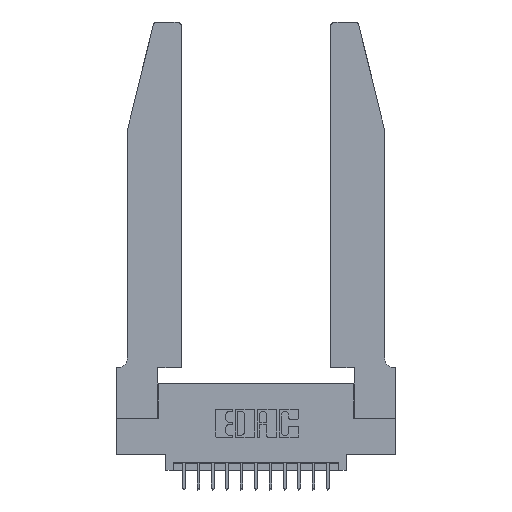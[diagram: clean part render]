
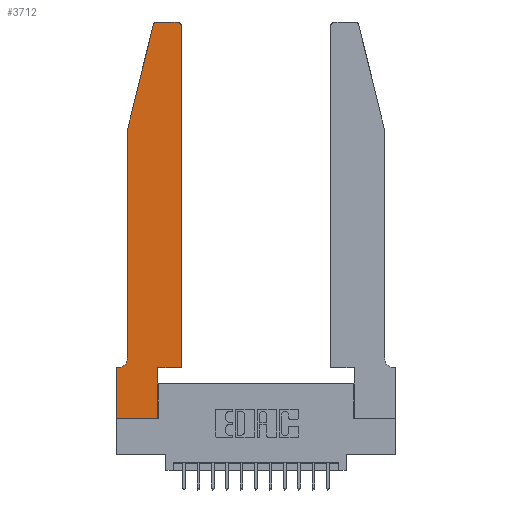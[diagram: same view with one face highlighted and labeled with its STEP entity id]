
A CAD part, top view. The second image highlights one B-rep face of the part: STEP entity #3712.
In plain terms, the highlighted planar face has unit normal (0, 0, 1).
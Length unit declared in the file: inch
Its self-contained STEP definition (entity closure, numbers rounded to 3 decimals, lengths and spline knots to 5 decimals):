
#22 = CARTESIAN_POINT ( 'NONE',  ( 0.284, 2.72, 0.37 ) ) ;
#60 = ORIENTED_EDGE ( 'NONE', *, *, #2111, .T. ) ;
#115 = CARTESIAN_POINT ( 'NONE',  ( 0.0755, 2., 0.37 ) ) ;
#117 = ORIENTED_EDGE ( 'NONE', *, *, #16556, .T. ) ;
#220 = CARTESIAN_POINT ( 'NONE',  ( 0.0055, 0.42, 0.37 ) ) ;
#293 = VERTEX_POINT ( 'NONE', #6411 ) ;
#375 = LINE ( 'NONE', #3556, #711 ) ;
#404 = ORIENTED_EDGE ( 'NONE', *, *, #10554, .T. ) ;
#443 = DIRECTION ( 'NONE',  ( 1., 0., 0. ) ) ;
#464 = EDGE_CURVE ( 'NONE', #1715, #6532, #1582, .T. ) ;
#477 = ORIENTED_EDGE ( 'NONE', *, *, #828, .T. ) ;
#711 = VECTOR ( 'NONE', #6002, 39.37008 ) ;
#828 = EDGE_CURVE ( 'NONE', #2811, #15147, #6665, .T. ) ;
#932 = VECTOR ( 'NONE', #8407, 39.37008 ) ;
#1094 = CARTESIAN_POINT ( 'NONE',  ( 0.0755, 0.42, 0.37 ) ) ;
#1474 = DIRECTION ( 'NONE',  ( 0., -1., 0. ) ) ;
#1496 = VERTEX_POINT ( 'NONE', #9986 ) ;
#1582 = LINE ( 'NONE', #15172, #8082 ) ;
#1639 = ORIENTED_EDGE ( 'NONE', *, *, #8259, .T. ) ;
#1715 = VERTEX_POINT ( 'NONE', #17118 ) ;
#1795 = CARTESIAN_POINT ( 'NONE',  ( 0.4205, 2.72, 0.37 ) ) ;
#2041 = EDGE_CURVE ( 'NONE', #10743, #7984, #7727, .T. ) ;
#2111 = EDGE_CURVE ( 'NONE', #1496, #2811, #12079, .T. ) ;
#2291 = DIRECTION ( 'NONE',  ( 0., 1., 0. ) ) ;
#2443 = CARTESIAN_POINT ( 'NONE',  ( 0.284, 2.75, 0.37 ) ) ;
#2573 = DIRECTION ( 'NONE',  ( 1., 0., 0. ) ) ;
#2596 = EDGE_CURVE ( 'NONE', #6532, #5245, #15212, .T. ) ;
#2781 = LINE ( 'NONE', #12208, #9853 ) ;
#2811 = VERTEX_POINT ( 'NONE', #2443 ) ;
#2890 = EDGE_CURVE ( 'NONE', #5245, #10743, #6313, .T. ) ;
#2916 = CARTESIAN_POINT ( 'NONE',  ( 0., 0., 0.37 ) ) ;
#3207 = ORIENTED_EDGE ( 'NONE', *, *, #2041, .T. ) ;
#3556 = CARTESIAN_POINT ( 'NONE',  ( 0.0755, 0.35, 0.37 ) ) ;
#3590 = DIRECTION ( 'NONE',  ( 1., 0., 0. ) ) ;
#3657 = CARTESIAN_POINT ( 'NONE',  ( 0.4505, 0.35, 0.37 ) ) ;
#3712 = ADVANCED_FACE ( 'NONE', ( #9360 ), #6315, .T. ) ;
#4215 = LINE ( 'NONE', #115, #12793 ) ;
#4245 = CARTESIAN_POINT ( 'NONE',  ( 0.2865, 0., 0.37 ) ) ;
#4260 = ORIENTED_EDGE ( 'NONE', *, *, #16723, .T. ) ;
#5245 = VERTEX_POINT ( 'NONE', #4245 ) ;
#5813 = DIRECTION ( 'NONE',  ( 0., -1., 0. ) ) ;
#5852 = VECTOR ( 'NONE', #13533, 39.37008 ) ;
#6002 = DIRECTION ( 'NONE',  ( -1., 0., 0. ) ) ;
#6084 = VERTEX_POINT ( 'NONE', #1094 ) ;
#6313 = LINE ( 'NONE', #7840, #6437 ) ;
#6315 = PLANE ( 'NONE',  #17601 ) ;
#6411 = CARTESIAN_POINT ( 'NONE',  ( 0.0755, 2., 0.37 ) ) ;
#6424 = ORIENTED_EDGE ( 'NONE', *, *, #2890, .T. ) ;
#6437 = VECTOR ( 'NONE', #14444, 39.37008 ) ;
#6532 = VERTEX_POINT ( 'NONE', #12898 ) ;
#6575 = EDGE_LOOP ( 'NONE', ( #60, #477, #404, #117, #8854, #4260, #8064, #16525, #6424, #3207, #1639, #16360 ) ) ;
#6665 = CIRCLE ( 'NONE', #10397, 0.03 ) ;
#6673 = CARTESIAN_POINT ( 'NONE',  ( 0.25487, 2.72718, 0.37 ) ) ;
#6822 = CARTESIAN_POINT ( 'NONE',  ( 0.2605, 2.75, 0.37 ) ) ;
#7135 = EDGE_CURVE ( 'NONE', #9509, #1496, #14598, .T. ) ;
#7508 = VECTOR ( 'NONE', #2291, 39.37008 ) ;
#7727 = LINE ( 'NONE', #11747, #15566 ) ;
#7840 = CARTESIAN_POINT ( 'NONE',  ( 0.2865, 0.35, 0.37 ) ) ;
#7984 = VERTEX_POINT ( 'NONE', #11941 ) ;
#8064 = ORIENTED_EDGE ( 'NONE', *, *, #464, .T. ) ;
#8082 = VECTOR ( 'NONE', #1474, 39.37008 ) ;
#8259 = EDGE_CURVE ( 'NONE', #7984, #9509, #10513, .T. ) ;
#8349 = VERTEX_POINT ( 'NONE', #16586 ) ;
#8407 = DIRECTION ( 'NONE',  ( 1., 0., 0. ) ) ;
#8408 = AXIS2_PLACEMENT_3D ( 'NONE', #220, #13648, #14997 ) ;
#8854 = ORIENTED_EDGE ( 'NONE', *, *, #12452, .T. ) ;
#9360 = FACE_OUTER_BOUND ( 'NONE', #6575, .T. ) ;
#9509 = VERTEX_POINT ( 'NONE', #16722 ) ;
#9853 = VECTOR ( 'NONE', #16422, 39.37008 ) ;
#9986 = CARTESIAN_POINT ( 'NONE',  ( 0.4205, 2.75, 0.37 ) ) ;
#10397 = AXIS2_PLACEMENT_3D ( 'NONE', #22, #17658, #2573 ) ;
#10513 = LINE ( 'NONE', #3657, #7508 ) ;
#10554 = EDGE_CURVE ( 'NONE', #15147, #293, #2781, .T. ) ;
#10743 = VERTEX_POINT ( 'NONE', #10866 ) ;
#10866 = CARTESIAN_POINT ( 'NONE',  ( 0.2865, 0.35, 0.37 ) ) ;
#11544 = CIRCLE ( 'NONE', #8408, 0.07 ) ;
#11747 = CARTESIAN_POINT ( 'NONE',  ( 0.4505, 0.35, 0.37 ) ) ;
#11941 = CARTESIAN_POINT ( 'NONE',  ( 0.4505, 0.35, 0.37 ) ) ;
#12079 = LINE ( 'NONE', #6822, #5852 ) ;
#12208 = CARTESIAN_POINT ( 'NONE',  ( 0.0755, 2., 0.37 ) ) ;
#12452 = EDGE_CURVE ( 'NONE', #6084, #8349, #11544, .T. ) ;
#12775 = DIRECTION ( 'NONE',  ( 0., 0., 1. ) ) ;
#12793 = VECTOR ( 'NONE', #5813, 39.37008 ) ;
#12897 = AXIS2_PLACEMENT_3D ( 'NONE', #1795, #12775, #443 ) ;
#12898 = CARTESIAN_POINT ( 'NONE',  ( 0., 0., 0.37 ) ) ;
#13533 = DIRECTION ( 'NONE',  ( -1., 0., 0. ) ) ;
#13648 = DIRECTION ( 'NONE',  ( 0., 0., -1. ) ) ;
#14444 = DIRECTION ( 'NONE',  ( 0., 1., 0. ) ) ;
#14598 = CIRCLE ( 'NONE', #12897, 0.03 ) ;
#14811 = CARTESIAN_POINT ( 'NONE',  ( 0., 0.35, 0.37 ) ) ;
#14997 = DIRECTION ( 'NONE',  ( -1., 0., 0. ) ) ;
#15147 = VERTEX_POINT ( 'NONE', #6673 ) ;
#15172 = CARTESIAN_POINT ( 'NONE',  ( 0., 0., 0.37 ) ) ;
#15212 = LINE ( 'NONE', #2916, #932 ) ;
#15566 = VECTOR ( 'NONE', #17231, 39.37008 ) ;
#16360 = ORIENTED_EDGE ( 'NONE', *, *, #7135, .T. ) ;
#16422 = DIRECTION ( 'NONE',  ( -0.239, -0.971, 0. ) ) ;
#16525 = ORIENTED_EDGE ( 'NONE', *, *, #2596, .T. ) ;
#16556 = EDGE_CURVE ( 'NONE', #293, #6084, #4215, .T. ) ;
#16586 = CARTESIAN_POINT ( 'NONE',  ( 0.0055, 0.35, 0.37 ) ) ;
#16722 = CARTESIAN_POINT ( 'NONE',  ( 0.4505, 2.72, 0.37 ) ) ;
#16723 = EDGE_CURVE ( 'NONE', #8349, #1715, #375, .T. ) ;
#17118 = CARTESIAN_POINT ( 'NONE',  ( 0., 0.35, 0.37 ) ) ;
#17231 = DIRECTION ( 'NONE',  ( 1., 0., 0. ) ) ;
#17333 = DIRECTION ( 'NONE',  ( 0., 0., 1. ) ) ;
#17601 = AXIS2_PLACEMENT_3D ( 'NONE', #14811, #17333, #3590 ) ;
#17658 = DIRECTION ( 'NONE',  ( 0., 0., 1. ) ) ;
